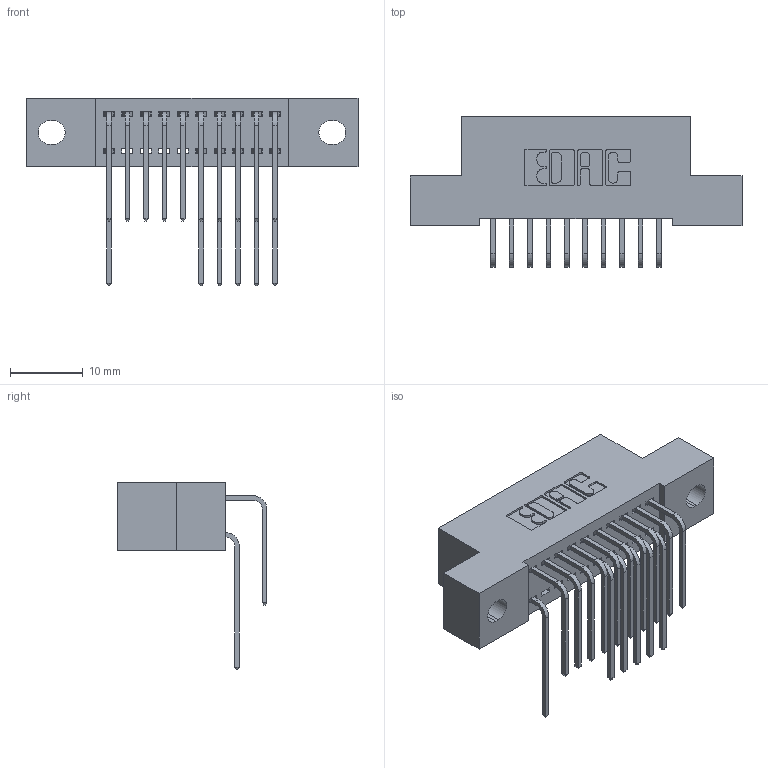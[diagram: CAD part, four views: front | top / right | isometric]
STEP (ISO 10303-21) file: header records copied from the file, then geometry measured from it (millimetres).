
FILE_DESCRIPTION (( 'STEP AP203' ), '1' );
FILE_NAME ('392-020-559-202.STEP', '2018-08-15T07:23:49', ( '' ), ( '' ), 'SwSTEP 2.0', 'SolidWorks 2016', '' );
FILE_SCHEMA (( 'CONFIG_CONTROL_DESIGN' ));
Length unit declared in the file: inch
Products named in the file (4): 345-292-001_558 559 Tail - 1; 345-292-001_559 Tail - 2; 392-020-559-202; 342 Part_.128 Slot
Assembly tree (17 placements, depth 2):
  392-020-559-202
    342 Part_.128 Slot
    345-292-001_558 559 Tail - 1  x6
    345-292-001_559 Tail - 2  x10
Bounding box: 45.72 x 20.64 x 25.78 mm (x, y, z)
Volume: 3960.6 mm3; surface area: 5636.5 mm2
Topology: 17 solids, 17 shells, 1002 faces, 2971 edges, 1958 vertices
Faces by surface type: plane 702, cylinder 300
Entity records: 12231 total; most frequent: CARTESIAN_POINT 2133, ORIENTED_EDGE 2022, DIRECTION 1855, EDGE_CURVE 1011, LINE 843, VECTOR 843, VERTEX_POINT 670, AXIS2_PLACEMENT_3D 506
